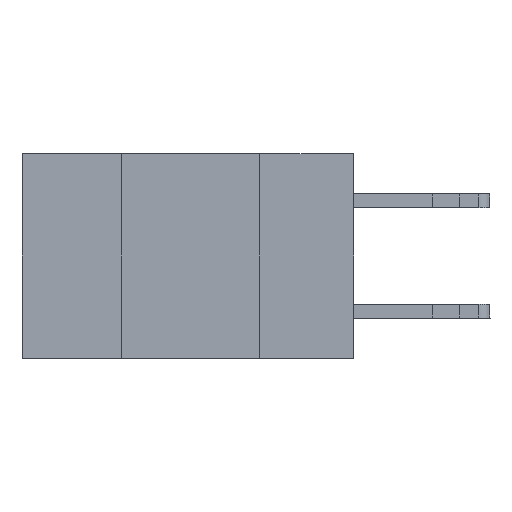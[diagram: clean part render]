
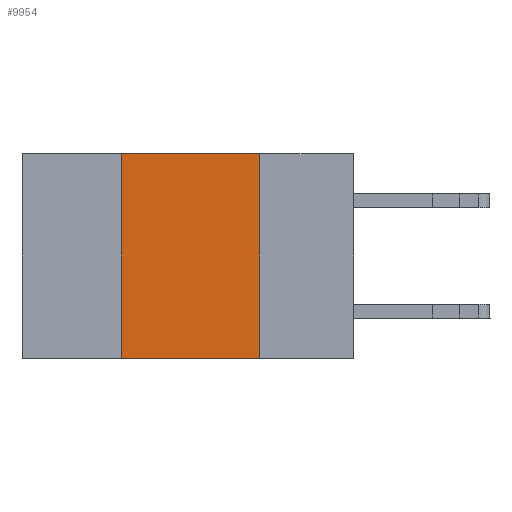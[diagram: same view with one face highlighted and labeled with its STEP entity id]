
A CAD part, left-side view. The second image highlights one B-rep face of the part: STEP entity #9954.
In plain terms, the highlighted planar face has unit normal (-1, 0, 0).
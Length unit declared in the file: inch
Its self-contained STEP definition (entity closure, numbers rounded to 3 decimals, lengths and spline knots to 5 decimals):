
#863 = VERTEX_POINT ( 'NONE', #3513 ) ;
#1202 = DIRECTION ( 'NONE',  ( 0., -1., 0. ) ) ;
#1554 = EDGE_CURVE ( 'NONE', #17677, #863, #17618, .T. ) ;
#2158 = LINE ( 'NONE', #18828, #18618 ) ;
#3489 = DIRECTION ( 'NONE',  ( 0., -1., 0. ) ) ;
#3513 = CARTESIAN_POINT ( 'NONE',  ( 0., 0.17, 0. ) ) ;
#3906 = EDGE_CURVE ( 'NONE', #15061, #17677, #16329, .T. ) ;
#4426 = EDGE_CURVE ( 'NONE', #15061, #15101, #10678, .T. ) ;
#5562 = CARTESIAN_POINT ( 'NONE',  ( 0., 0.42, -0.37 ) ) ;
#5748 = DIRECTION ( 'NONE',  ( 0., 0., -1. ) ) ;
#6061 = CARTESIAN_POINT ( 'NONE',  ( 0., 0.6, -0.37 ) ) ;
#9374 = FACE_OUTER_BOUND ( 'NONE', #9757, .T. ) ;
#9610 = CARTESIAN_POINT ( 'NONE',  ( 0., 0.6, 0. ) ) ;
#9757 = EDGE_LOOP ( 'NONE', ( #19738, #12050, #16180, #16674 ) ) ;
#9954 = ADVANCED_FACE ( 'NONE', ( #9374 ), #13760, .F. ) ;
#10678 = LINE ( 'NONE', #6061, #18489 ) ;
#11078 = DIRECTION ( 'NONE',  ( 0., 0., -1. ) ) ;
#12050 = ORIENTED_EDGE ( 'NONE', *, *, #1554, .F. ) ;
#12190 = CARTESIAN_POINT ( 'NONE',  ( 0., 0.6, 0. ) ) ;
#12217 = VECTOR ( 'NONE', #15983, 39.37008 ) ;
#12849 = CARTESIAN_POINT ( 'NONE',  ( 0., 0.42, 0. ) ) ;
#13076 = CARTESIAN_POINT ( 'NONE',  ( 0., 0.42, 0. ) ) ;
#13503 = VECTOR ( 'NONE', #3489, 39.37008 ) ;
#13760 = PLANE ( 'NONE',  #14927 ) ;
#14927 = AXIS2_PLACEMENT_3D ( 'NONE', #12190, #15309, #5748 ) ;
#15061 = VERTEX_POINT ( 'NONE', #5562 ) ;
#15101 = VERTEX_POINT ( 'NONE', #15135 ) ;
#15135 = CARTESIAN_POINT ( 'NONE',  ( 0., 0.17, -0.37 ) ) ;
#15309 = DIRECTION ( 'NONE',  ( 1., 0., 0. ) ) ;
#15983 = DIRECTION ( 'NONE',  ( 0., 0., 1. ) ) ;
#16180 = ORIENTED_EDGE ( 'NONE', *, *, #3906, .F. ) ;
#16329 = LINE ( 'NONE', #12849, #12217 ) ;
#16674 = ORIENTED_EDGE ( 'NONE', *, *, #4426, .T. ) ;
#17618 = LINE ( 'NONE', #9610, #13503 ) ;
#17677 = VERTEX_POINT ( 'NONE', #13076 ) ;
#18489 = VECTOR ( 'NONE', #1202, 39.37008 ) ;
#18618 = VECTOR ( 'NONE', #11078, 39.37008 ) ;
#18828 = CARTESIAN_POINT ( 'NONE',  ( 0., 0.17, 0. ) ) ;
#19738 = ORIENTED_EDGE ( 'NONE', *, *, #20289, .F. ) ;
#20289 = EDGE_CURVE ( 'NONE', #863, #15101, #2158, .T. ) ;
